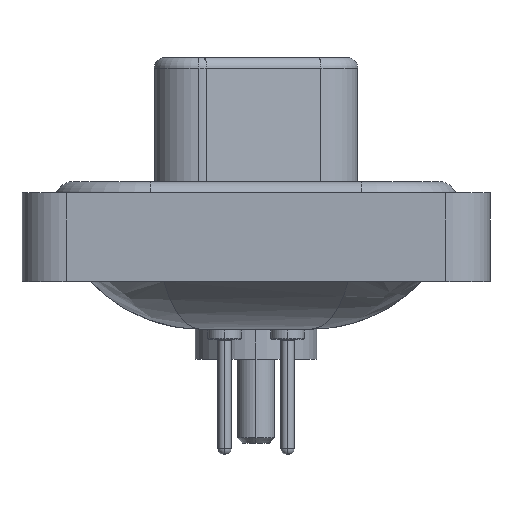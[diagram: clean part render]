
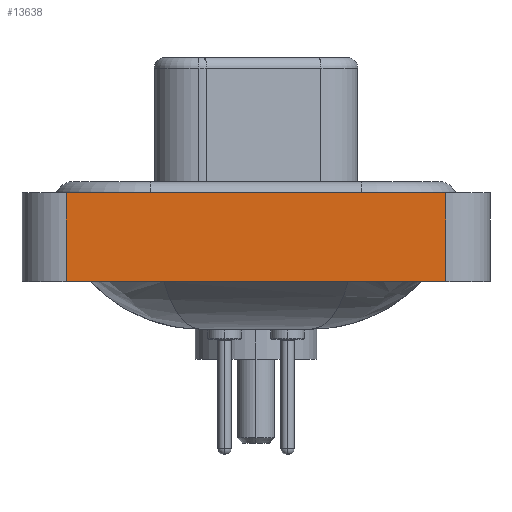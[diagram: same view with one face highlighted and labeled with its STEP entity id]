
A CAD part, left-side view. The second image highlights one B-rep face of the part: STEP entity #13638.
In plain terms, the highlighted planar face has unit normal (-1, 0, 0).
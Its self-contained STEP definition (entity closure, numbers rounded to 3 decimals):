
#280 = EDGE_CURVE ( 'NONE', #12933, #21846, #13630, .T. ) ;
#352 = DIRECTION ( 'NONE',  ( -1., 0., 0. ) ) ;
#1740 = LINE ( 'NONE', #18762, #20138 ) ;
#2444 = VERTEX_POINT ( 'NONE', #3072 ) ;
#3010 = CARTESIAN_POINT ( 'NONE',  ( -7.35, 8.55, -3.6 ) ) ;
#3072 = CARTESIAN_POINT ( 'NONE',  ( -7.35, -8.55, 0.4 ) ) ;
#3664 = VERTEX_POINT ( 'NONE', #10043 ) ;
#4468 = CARTESIAN_POINT ( 'NONE',  ( -7.35, -8.55, -3.6 ) ) ;
#4610 = DIRECTION ( 'NONE',  ( 0., 0., 1. ) ) ;
#5823 = DIRECTION ( 'NONE',  ( 0., 0., 1. ) ) ;
#6446 = DIRECTION ( 'NONE',  ( 0., -1., 0. ) ) ;
#8570 = LINE ( 'NONE', #18410, #20205 ) ;
#9049 = DIRECTION ( 'NONE',  ( 0., 0., 1. ) ) ;
#9106 = VECTOR ( 'NONE', #6446, 1000. ) ;
#9529 = AXIS2_PLACEMENT_3D ( 'NONE', #4468, #352, #5823 ) ;
#9688 = EDGE_CURVE ( 'NONE', #12933, #3664, #8570, .T. ) ;
#10043 = CARTESIAN_POINT ( 'NONE',  ( -7.35, -8.55, -3.6 ) ) ;
#12933 = VERTEX_POINT ( 'NONE', #3010 ) ;
#13580 = EDGE_CURVE ( 'NONE', #3664, #2444, #1740, .T. ) ;
#13630 = LINE ( 'NONE', #14001, #22861 ) ;
#13638 = ADVANCED_FACE ( 'NONE', ( #17523 ), #15211, .T. ) ;
#14001 = CARTESIAN_POINT ( 'NONE',  ( -7.35, 8.55, -3.6 ) ) ;
#14153 = ORIENTED_EDGE ( 'NONE', *, *, #13580, .T. ) ;
#15160 = EDGE_CURVE ( 'NONE', #21846, #2444, #15322, .T. ) ;
#15211 = PLANE ( 'NONE',  #9529 ) ;
#15312 = EDGE_LOOP ( 'NONE', ( #14153, #15565, #19002, #17525 ) ) ;
#15322 = LINE ( 'NONE', #23075, #9106 ) ;
#15565 = ORIENTED_EDGE ( 'NONE', *, *, #15160, .F. ) ;
#17523 = FACE_OUTER_BOUND ( 'NONE', #15312, .T. ) ;
#17525 = ORIENTED_EDGE ( 'NONE', *, *, #9688, .T. ) ;
#18165 = DIRECTION ( 'NONE',  ( 0., -1., 0. ) ) ;
#18410 = CARTESIAN_POINT ( 'NONE',  ( -7.35, -8.55, -3.6 ) ) ;
#18762 = CARTESIAN_POINT ( 'NONE',  ( -7.35, -8.55, -3.6 ) ) ;
#19002 = ORIENTED_EDGE ( 'NONE', *, *, #280, .F. ) ;
#20138 = VECTOR ( 'NONE', #9049, 1000. ) ;
#20205 = VECTOR ( 'NONE', #18165, 1000. ) ;
#21225 = CARTESIAN_POINT ( 'NONE',  ( -7.35, 8.55, 0.4 ) ) ;
#21846 = VERTEX_POINT ( 'NONE', #21225 ) ;
#22861 = VECTOR ( 'NONE', #4610, 1000. ) ;
#23075 = CARTESIAN_POINT ( 'NONE',  ( -7.35, -8.55, 0.4 ) ) ;
